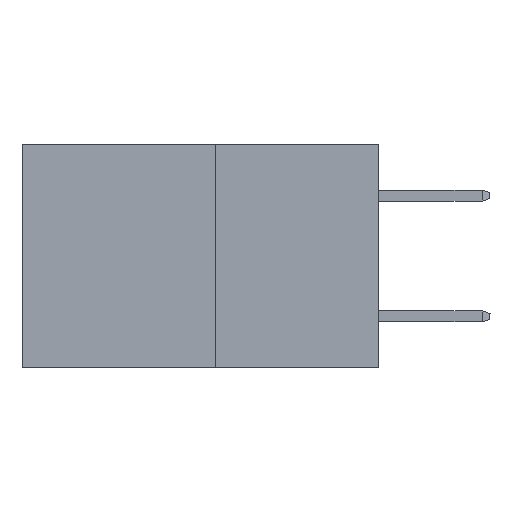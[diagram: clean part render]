
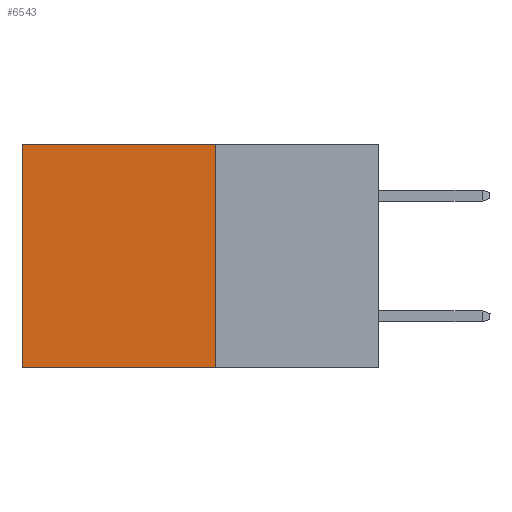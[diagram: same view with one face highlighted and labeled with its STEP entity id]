
A CAD part, left-side view. The second image highlights one B-rep face of the part: STEP entity #6543.
In plain terms, the highlighted planar face has unit normal (-1, 0, 0).
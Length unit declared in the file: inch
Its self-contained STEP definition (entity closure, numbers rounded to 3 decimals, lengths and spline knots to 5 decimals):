
#380 = LINE ( 'NONE', #3114, #5332 ) ;
#779 = CARTESIAN_POINT ( 'NONE',  ( 0.277, 0.27, -0.37 ) ) ;
#1508 = EDGE_CURVE ( 'NONE', #4488, #4581, #380, .T. ) ;
#1912 = AXIS2_PLACEMENT_3D ( 'NONE', #779, #4755, #10613 ) ;
#2329 = CARTESIAN_POINT ( 'NONE',  ( 0.277, 0.59, -0.37 ) ) ;
#2896 = EDGE_CURVE ( 'NONE', #4488, #7642, #10001, .T. ) ;
#2928 = ORIENTED_EDGE ( 'NONE', *, *, #7152, .F. ) ;
#3038 = VECTOR ( 'NONE', #10136, 39.37008 ) ;
#3114 = CARTESIAN_POINT ( 'NONE',  ( 0.277, 0.27, -0.37 ) ) ;
#3427 = LINE ( 'NONE', #2329, #3746 ) ;
#3440 = ORIENTED_EDGE ( 'NONE', *, *, #1508, .F. ) ;
#3746 = VECTOR ( 'NONE', #8594, 39.37008 ) ;
#4144 = CARTESIAN_POINT ( 'NONE',  ( 0.277, 0.59, 0. ) ) ;
#4488 = VERTEX_POINT ( 'NONE', #8097 ) ;
#4581 = VERTEX_POINT ( 'NONE', #6427 ) ;
#4737 = CARTESIAN_POINT ( 'NONE',  ( 0.277, 0.59, -0.37 ) ) ;
#4755 = DIRECTION ( 'NONE',  ( 1., 0., 0. ) ) ;
#5332 = VECTOR ( 'NONE', #10002, 39.37008 ) ;
#5482 = DIRECTION ( 'NONE',  ( 0., 1., 0. ) ) ;
#5661 = VECTOR ( 'NONE', #5482, 39.37008 ) ;
#5932 = LINE ( 'NONE', #8837, #5661 ) ;
#6188 = FACE_OUTER_BOUND ( 'NONE', #8253, .T. ) ;
#6427 = CARTESIAN_POINT ( 'NONE',  ( 0.277, 0.27, -0.37 ) ) ;
#6543 = ADVANCED_FACE ( 'NONE', ( #6188 ), #9803, .F. ) ;
#7030 = ORIENTED_EDGE ( 'NONE', *, *, #2896, .T. ) ;
#7138 = ORIENTED_EDGE ( 'NONE', *, *, #8698, .T. ) ;
#7152 = EDGE_CURVE ( 'NONE', #4581, #10672, #5932, .T. ) ;
#7642 = VERTEX_POINT ( 'NONE', #4144 ) ;
#7684 = CARTESIAN_POINT ( 'NONE',  ( 0.277, 0.27, 0. ) ) ;
#8097 = CARTESIAN_POINT ( 'NONE',  ( 0.277, 0.27, 0. ) ) ;
#8253 = EDGE_LOOP ( 'NONE', ( #7138, #2928, #3440, #7030 ) ) ;
#8594 = DIRECTION ( 'NONE',  ( 0., 0., -1. ) ) ;
#8698 = EDGE_CURVE ( 'NONE', #7642, #10672, #3427, .T. ) ;
#8837 = CARTESIAN_POINT ( 'NONE',  ( 0.277, 0.27, -0.37 ) ) ;
#9803 = PLANE ( 'NONE',  #1912 ) ;
#10001 = LINE ( 'NONE', #7684, #3038 ) ;
#10002 = DIRECTION ( 'NONE',  ( 0., 0., -1. ) ) ;
#10136 = DIRECTION ( 'NONE',  ( 0., 1., 0. ) ) ;
#10613 = DIRECTION ( 'NONE',  ( 0., 0., -1. ) ) ;
#10672 = VERTEX_POINT ( 'NONE', #4737 ) ;
